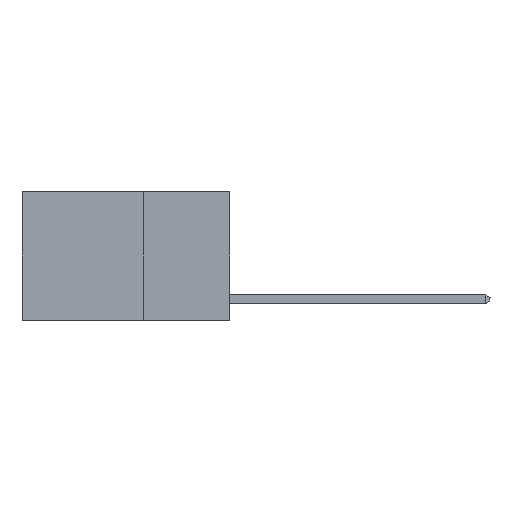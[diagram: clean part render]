
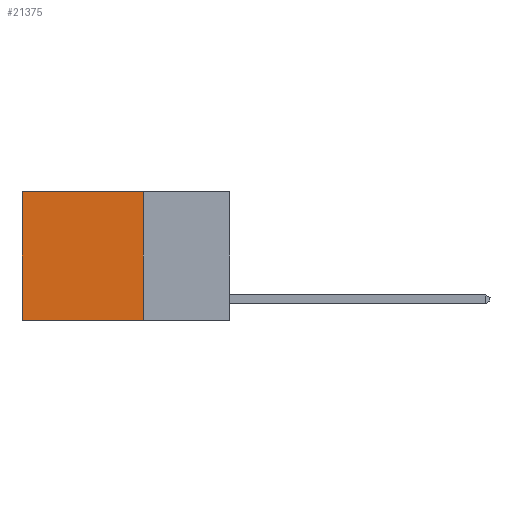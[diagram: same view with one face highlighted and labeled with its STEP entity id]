
A CAD part, left-side view. The second image highlights one B-rep face of the part: STEP entity #21375.
In plain terms, the highlighted planar face has unit normal (-1, 0, 0).
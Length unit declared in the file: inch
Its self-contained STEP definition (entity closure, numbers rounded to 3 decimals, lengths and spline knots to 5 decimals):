
#5 = DIRECTION ( 'NONE',  ( 1., 0., 0. ) ) ;
#256 = LINE ( 'NONE', #384, #7685 ) ;
#384 = CARTESIAN_POINT ( 'NONE',  ( 0.2625, 0.6, 0. ) ) ;
#614 = VECTOR ( 'NONE', #14638, 39.37008 ) ;
#1269 = VECTOR ( 'NONE', #22727, 39.37008 ) ;
#2191 = CARTESIAN_POINT ( 'NONE',  ( 0.2625, 0.25, 0. ) ) ;
#2723 = LINE ( 'NONE', #8262, #614 ) ;
#3063 = LINE ( 'NONE', #22702, #11775 ) ;
#3641 = VERTEX_POINT ( 'NONE', #6989 ) ;
#4559 = LINE ( 'NONE', #10820, #1269 ) ;
#4878 = EDGE_CURVE ( 'NONE', #3641, #18961, #4559, .T. ) ;
#5312 = ORIENTED_EDGE ( 'NONE', *, *, #23538, .F. ) ;
#6022 = VERTEX_POINT ( 'NONE', #15433 ) ;
#6253 = DIRECTION ( 'NONE',  ( 0., 0., -1. ) ) ;
#6989 = CARTESIAN_POINT ( 'NONE',  ( 0.2625, 0.25, 0. ) ) ;
#7685 = VECTOR ( 'NONE', #6253, 39.37008 ) ;
#8262 = CARTESIAN_POINT ( 'NONE',  ( 0.2625, 0.25, 0. ) ) ;
#9273 = CARTESIAN_POINT ( 'NONE',  ( 0.2625, 0.25, -0.37 ) ) ;
#10091 = ORIENTED_EDGE ( 'NONE', *, *, #4878, .T. ) ;
#10820 = CARTESIAN_POINT ( 'NONE',  ( 0.2625, 0.25, 0. ) ) ;
#11189 = AXIS2_PLACEMENT_3D ( 'NONE', #2191, #5, #12016 ) ;
#11775 = VECTOR ( 'NONE', #16936, 39.37008 ) ;
#12016 = DIRECTION ( 'NONE',  ( 0., 0., -1. ) ) ;
#12812 = EDGE_CURVE ( 'NONE', #18961, #6022, #256, .T. ) ;
#13699 = EDGE_CURVE ( 'NONE', #3641, #17863, #2723, .T. ) ;
#14108 = FACE_OUTER_BOUND ( 'NONE', #20753, .T. ) ;
#14561 = CARTESIAN_POINT ( 'NONE',  ( 0.2625, 0.6, 0. ) ) ;
#14638 = DIRECTION ( 'NONE',  ( 0., 0., -1. ) ) ;
#15433 = CARTESIAN_POINT ( 'NONE',  ( 0.2625, 0.6, -0.37 ) ) ;
#16467 = ORIENTED_EDGE ( 'NONE', *, *, #13699, .F. ) ;
#16936 = DIRECTION ( 'NONE',  ( 0., 1., 0. ) ) ;
#17863 = VERTEX_POINT ( 'NONE', #9273 ) ;
#18961 = VERTEX_POINT ( 'NONE', #14561 ) ;
#20753 = EDGE_LOOP ( 'NONE', ( #23624, #5312, #16467, #10091 ) ) ;
#21375 = ADVANCED_FACE ( 'NONE', ( #14108 ), #23920, .F. ) ;
#22702 = CARTESIAN_POINT ( 'NONE',  ( 0.2625, 0.25, -0.37 ) ) ;
#22727 = DIRECTION ( 'NONE',  ( 0., 1., 0. ) ) ;
#23538 = EDGE_CURVE ( 'NONE', #17863, #6022, #3063, .T. ) ;
#23624 = ORIENTED_EDGE ( 'NONE', *, *, #12812, .T. ) ;
#23920 = PLANE ( 'NONE',  #11189 ) ;
